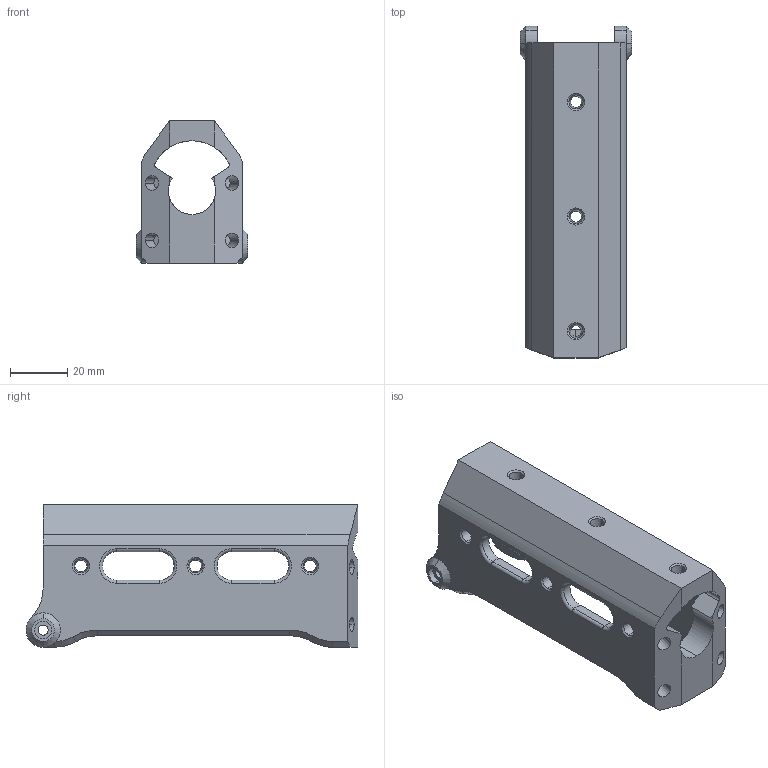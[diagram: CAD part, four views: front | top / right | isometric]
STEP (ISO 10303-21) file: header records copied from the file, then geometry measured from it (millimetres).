
FILE_DESCRIPTION (( 'STEP AP214' ), '1' );
FILE_NAME ('Frame_Shroud_V10.STEP', '2025-07-07T03:52:04', ( '' ), ( '' ), 'SwSTEP 2.0', 'SolidWorks 2020', '' );
FILE_SCHEMA (( 'AUTOMOTIVE_DESIGN' ));
Length unit declared in the file: millimetre
Products named in the file (1): Frame_Shroud_V10
Bounding box: 39 x 115.89 x 49.75 mm (x, y, z)
Volume: 55340.5 mm3; surface area: 26363.8 mm2
Topology: 1 solids, 1 shells, 166 faces, 430 edges, 269 vertices
Faces by surface type: cone 59, plane 48, cylinder 45, torus 8, bspline 6
Entity records: 8451 total; most frequent: CARTESIAN_POINT 4259, DIRECTION 891, ORIENTED_EDGE 860, EDGE_CURVE 430, AXIS2_PLACEMENT_3D 343, VERTEX_POINT 269, LINE 205, VECTOR 205
